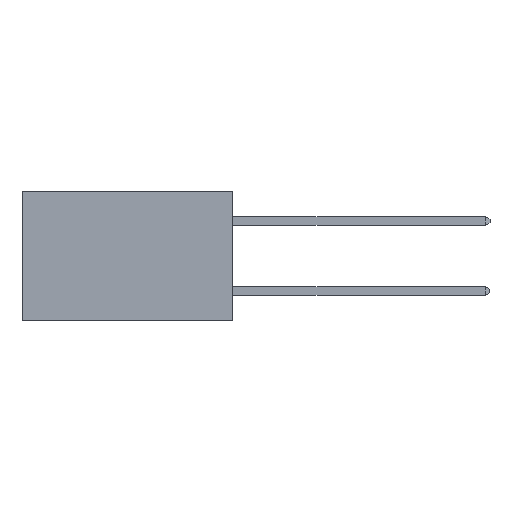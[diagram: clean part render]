
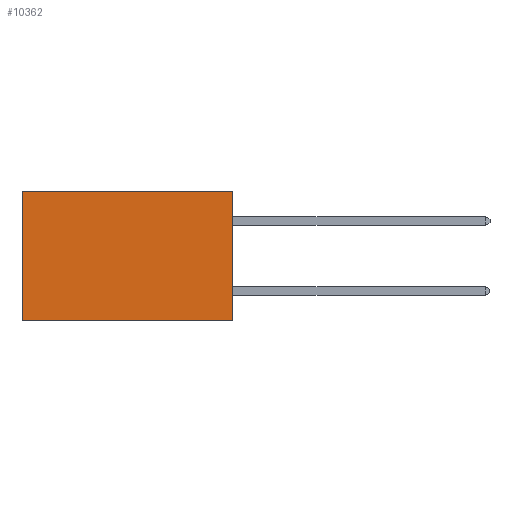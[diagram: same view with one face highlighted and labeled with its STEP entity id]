
A CAD part, left-side view. The second image highlights one B-rep face of the part: STEP entity #10362.
In plain terms, the highlighted planar face has unit normal (-1, 0, 0).
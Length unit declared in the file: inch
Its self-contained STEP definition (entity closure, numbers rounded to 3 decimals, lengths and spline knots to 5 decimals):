
#405 = VERTEX_POINT ( 'NONE', #4471 ) ;
#844 = DIRECTION ( 'NONE',  ( 1., 0., 0. ) ) ;
#1110 = VECTOR ( 'NONE', #7552, 39.37008 ) ;
#1595 = FACE_OUTER_BOUND ( 'NONE', #3818, .T. ) ;
#1773 = ORIENTED_EDGE ( 'NONE', *, *, #6170, .T. ) ;
#2380 = ORIENTED_EDGE ( 'NONE', *, *, #9488, .F. ) ;
#3006 = LINE ( 'NONE', #7570, #1110 ) ;
#3609 = AXIS2_PLACEMENT_3D ( 'NONE', #4901, #844, #6487 ) ;
#3762 = CARTESIAN_POINT ( 'NONE',  ( 0.2875, 0., -0.37 ) ) ;
#3818 = EDGE_LOOP ( 'NONE', ( #1773, #2380, #4588, #8698 ) ) ;
#4349 = VERTEX_POINT ( 'NONE', #8600 ) ;
#4417 = EDGE_CURVE ( 'NONE', #4349, #8555, #3006, .T. ) ;
#4471 = CARTESIAN_POINT ( 'NONE',  ( 0.2875, 0.6, 0. ) ) ;
#4588 = ORIENTED_EDGE ( 'NONE', *, *, #4417, .F. ) ;
#4901 = CARTESIAN_POINT ( 'NONE',  ( 0.2875, 0., 0. ) ) ;
#4975 = CARTESIAN_POINT ( 'NONE',  ( 0.2875, 0.6, 0. ) ) ;
#5260 = CARTESIAN_POINT ( 'NONE',  ( 0.2875, 0.6, -0.37 ) ) ;
#5314 = VECTOR ( 'NONE', #7363, 39.37008 ) ;
#5877 = DIRECTION ( 'NONE',  ( 0., 1., 0. ) ) ;
#6170 = EDGE_CURVE ( 'NONE', #405, #7979, #9646, .T. ) ;
#6487 = DIRECTION ( 'NONE',  ( 0., 0., -1. ) ) ;
#6884 = CARTESIAN_POINT ( 'NONE',  ( 0.2875, 0., -0.37 ) ) ;
#7017 = VECTOR ( 'NONE', #5877, 39.37008 ) ;
#7363 = DIRECTION ( 'NONE',  ( 0., 0., -1. ) ) ;
#7552 = DIRECTION ( 'NONE',  ( 0., 0., -1. ) ) ;
#7570 = CARTESIAN_POINT ( 'NONE',  ( 0.2875, 0., 0. ) ) ;
#7829 = EDGE_CURVE ( 'NONE', #4349, #405, #9463, .T. ) ;
#7951 = LINE ( 'NONE', #3762, #10184 ) ;
#7979 = VERTEX_POINT ( 'NONE', #5260 ) ;
#8555 = VERTEX_POINT ( 'NONE', #6884 ) ;
#8600 = CARTESIAN_POINT ( 'NONE',  ( 0.2875, 0., 0. ) ) ;
#8698 = ORIENTED_EDGE ( 'NONE', *, *, #7829, .T. ) ;
#9424 = DIRECTION ( 'NONE',  ( 0., 1., 0. ) ) ;
#9463 = LINE ( 'NONE', #9950, #7017 ) ;
#9488 = EDGE_CURVE ( 'NONE', #8555, #7979, #7951, .T. ) ;
#9646 = LINE ( 'NONE', #4975, #5314 ) ;
#9950 = CARTESIAN_POINT ( 'NONE',  ( 0.2875, 0., 0. ) ) ;
#10184 = VECTOR ( 'NONE', #9424, 39.37008 ) ;
#10362 = ADVANCED_FACE ( 'NONE', ( #1595 ), #10569, .F. ) ;
#10569 = PLANE ( 'NONE',  #3609 ) ;
